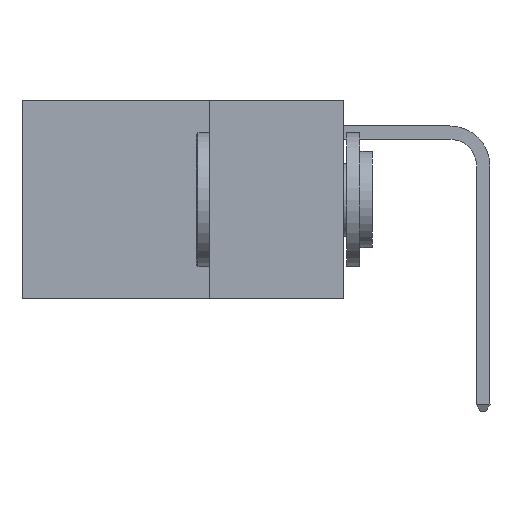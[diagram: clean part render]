
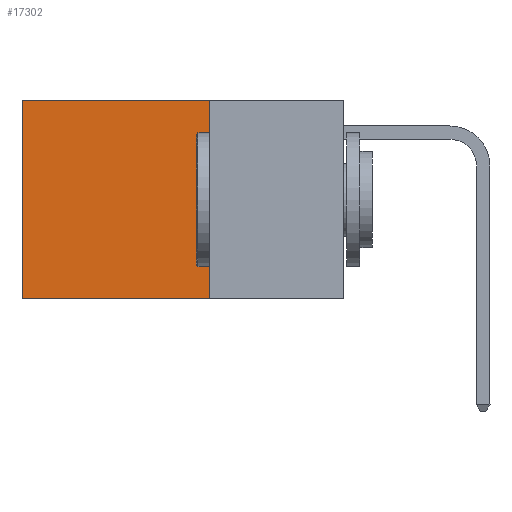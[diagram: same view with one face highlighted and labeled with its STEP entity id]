
A CAD part, left-side view. The second image highlights one B-rep face of the part: STEP entity #17302.
In plain terms, the highlighted planar face has unit normal (-1, 0, 0).
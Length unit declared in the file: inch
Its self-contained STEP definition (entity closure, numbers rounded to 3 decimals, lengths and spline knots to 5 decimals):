
#177 = ORIENTED_EDGE ( 'NONE', *, *, #3596, .F. ) ;
#370 = CARTESIAN_POINT ( 'NONE',  ( 0.2625, 0.25, 0. ) ) ;
#827 = VERTEX_POINT ( 'NONE', #18882 ) ;
#1795 = VERTEX_POINT ( 'NONE', #6897 ) ;
#2676 = AXIS2_PLACEMENT_3D ( 'NONE', #9478, #4358, #20548 ) ;
#3596 = EDGE_CURVE ( 'NONE', #21699, #1795, #17012, .T. ) ;
#4358 = DIRECTION ( 'NONE',  ( 1., 0., 0. ) ) ;
#4670 = LINE ( 'NONE', #6197, #11264 ) ;
#4727 = ORIENTED_EDGE ( 'NONE', *, *, #11121, .F. ) ;
#5239 = VECTOR ( 'NONE', #21209, 39.37008 ) ;
#6197 = CARTESIAN_POINT ( 'NONE',  ( 0.2625, 0.6, 0. ) ) ;
#6590 = EDGE_CURVE ( 'NONE', #827, #1795, #4670, .T. ) ;
#6664 = LINE ( 'NONE', #10591, #7270 ) ;
#6897 = CARTESIAN_POINT ( 'NONE',  ( 0.2625, 0.6, -0.37 ) ) ;
#7270 = VECTOR ( 'NONE', #20761, 39.37008 ) ;
#8012 = EDGE_CURVE ( 'NONE', #22367, #827, #8830, .T. ) ;
#8830 = LINE ( 'NONE', #370, #5239 ) ;
#8928 = ORIENTED_EDGE ( 'NONE', *, *, #8012, .T. ) ;
#9478 = CARTESIAN_POINT ( 'NONE',  ( 0.2625, 0.25, 0. ) ) ;
#10168 = DIRECTION ( 'NONE',  ( 0., 1., 0. ) ) ;
#10591 = CARTESIAN_POINT ( 'NONE',  ( 0.2625, 0.25, 0. ) ) ;
#11121 = EDGE_CURVE ( 'NONE', #22367, #21699, #6664, .T. ) ;
#11210 = VECTOR ( 'NONE', #10168, 39.37008 ) ;
#11264 = VECTOR ( 'NONE', #16631, 39.37008 ) ;
#13039 = FACE_OUTER_BOUND ( 'NONE', #16617, .T. ) ;
#14225 = CARTESIAN_POINT ( 'NONE',  ( 0.2625, 0.25, 0. ) ) ;
#16617 = EDGE_LOOP ( 'NONE', ( #20011, #177, #4727, #8928 ) ) ;
#16631 = DIRECTION ( 'NONE',  ( 0., 0., -1. ) ) ;
#16780 = CARTESIAN_POINT ( 'NONE',  ( 0.2625, 0.25, -0.37 ) ) ;
#17012 = LINE ( 'NONE', #16780, #11210 ) ;
#17302 = ADVANCED_FACE ( 'NONE', ( #13039 ), #18493, .F. ) ;
#17998 = CARTESIAN_POINT ( 'NONE',  ( 0.2625, 0.25, -0.37 ) ) ;
#18493 = PLANE ( 'NONE',  #2676 ) ;
#18882 = CARTESIAN_POINT ( 'NONE',  ( 0.2625, 0.6, 0. ) ) ;
#20011 = ORIENTED_EDGE ( 'NONE', *, *, #6590, .T. ) ;
#20548 = DIRECTION ( 'NONE',  ( 0., 0., -1. ) ) ;
#20761 = DIRECTION ( 'NONE',  ( 0., 0., -1. ) ) ;
#21209 = DIRECTION ( 'NONE',  ( 0., 1., 0. ) ) ;
#21699 = VERTEX_POINT ( 'NONE', #17998 ) ;
#22367 = VERTEX_POINT ( 'NONE', #14225 ) ;
